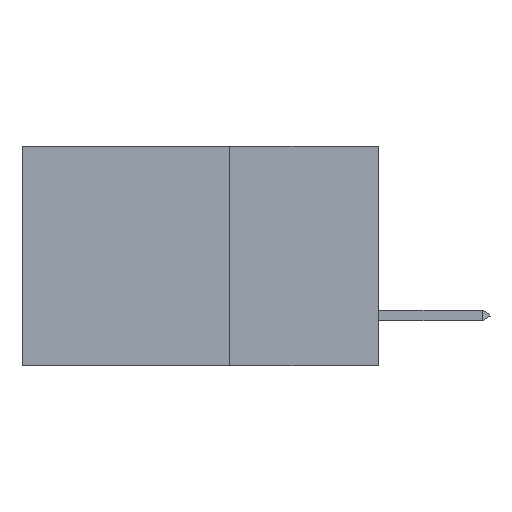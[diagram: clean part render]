
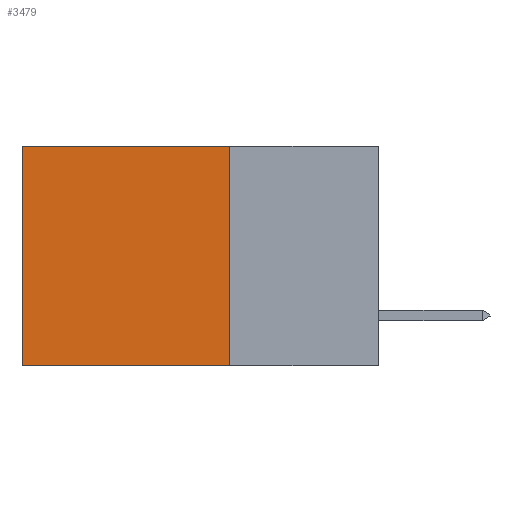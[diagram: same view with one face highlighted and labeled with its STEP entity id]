
A CAD part, left-side view. The second image highlights one B-rep face of the part: STEP entity #3479.
In plain terms, the highlighted planar face has unit normal (-1, 0, 0).
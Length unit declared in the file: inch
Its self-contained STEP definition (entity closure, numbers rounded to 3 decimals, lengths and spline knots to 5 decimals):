
#311 = ORIENTED_EDGE ( 'NONE', *, *, #11470, .T. ) ;
#690 = CARTESIAN_POINT ( 'NONE',  ( 0.298, 0.25, 0. ) ) ;
#1508 = ORIENTED_EDGE ( 'NONE', *, *, #2415, .F. ) ;
#1650 = DIRECTION ( 'NONE',  ( 0., 0., -1. ) ) ;
#2359 = VECTOR ( 'NONE', #8418, 39.37008 ) ;
#2415 = EDGE_CURVE ( 'NONE', #8746, #11930, #13294, .T. ) ;
#2837 = CARTESIAN_POINT ( 'NONE',  ( 0.298, 0.25, 0. ) ) ;
#3351 = VECTOR ( 'NONE', #11222, 39.37008 ) ;
#3479 = ADVANCED_FACE ( 'NONE', ( #5907 ), #8239, .F. ) ;
#3672 = ORIENTED_EDGE ( 'NONE', *, *, #13189, .T. ) ;
#4754 = VERTEX_POINT ( 'NONE', #8244 ) ;
#5431 = VERTEX_POINT ( 'NONE', #10992 ) ;
#5907 = FACE_OUTER_BOUND ( 'NONE', #6012, .T. ) ;
#6012 = EDGE_LOOP ( 'NONE', ( #3672, #1508, #8621, #311 ) ) ;
#7816 = CARTESIAN_POINT ( 'NONE',  ( 0.298, 0.6, 0. ) ) ;
#8239 = PLANE ( 'NONE',  #12504 ) ;
#8244 = CARTESIAN_POINT ( 'NONE',  ( 0.298, 0.25, 0. ) ) ;
#8418 = DIRECTION ( 'NONE',  ( 0., 1., 0. ) ) ;
#8618 = CARTESIAN_POINT ( 'NONE',  ( 0.298, 0.25, -0.37 ) ) ;
#8621 = ORIENTED_EDGE ( 'NONE', *, *, #11684, .F. ) ;
#8746 = VERTEX_POINT ( 'NONE', #11995 ) ;
#8891 = VECTOR ( 'NONE', #12841, 39.37008 ) ;
#9214 = LINE ( 'NONE', #7816, #3351 ) ;
#9226 = DIRECTION ( 'NONE',  ( 1., 0., 0. ) ) ;
#9919 = DIRECTION ( 'NONE',  ( 0., 1., 0. ) ) ;
#10260 = LINE ( 'NONE', #690, #8891 ) ;
#10992 = CARTESIAN_POINT ( 'NONE',  ( 0.298, 0.6, 0. ) ) ;
#11222 = DIRECTION ( 'NONE',  ( 0., 0., -1. ) ) ;
#11470 = EDGE_CURVE ( 'NONE', #4754, #5431, #11632, .T. ) ;
#11632 = LINE ( 'NONE', #2837, #2359 ) ;
#11684 = EDGE_CURVE ( 'NONE', #4754, #8746, #10260, .T. ) ;
#11930 = VERTEX_POINT ( 'NONE', #13587 ) ;
#11995 = CARTESIAN_POINT ( 'NONE',  ( 0.298, 0.25, -0.37 ) ) ;
#12109 = VECTOR ( 'NONE', #9919, 39.37008 ) ;
#12504 = AXIS2_PLACEMENT_3D ( 'NONE', #13651, #9226, #1650 ) ;
#12841 = DIRECTION ( 'NONE',  ( 0., 0., -1. ) ) ;
#13189 = EDGE_CURVE ( 'NONE', #5431, #11930, #9214, .T. ) ;
#13294 = LINE ( 'NONE', #8618, #12109 ) ;
#13587 = CARTESIAN_POINT ( 'NONE',  ( 0.298, 0.6, -0.37 ) ) ;
#13651 = CARTESIAN_POINT ( 'NONE',  ( 0.298, 0.25, 0. ) ) ;
